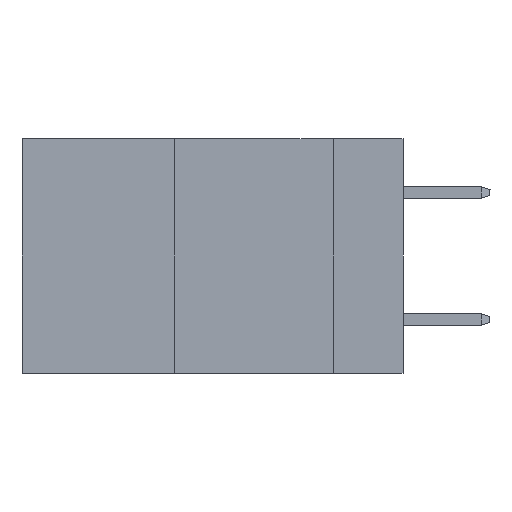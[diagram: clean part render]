
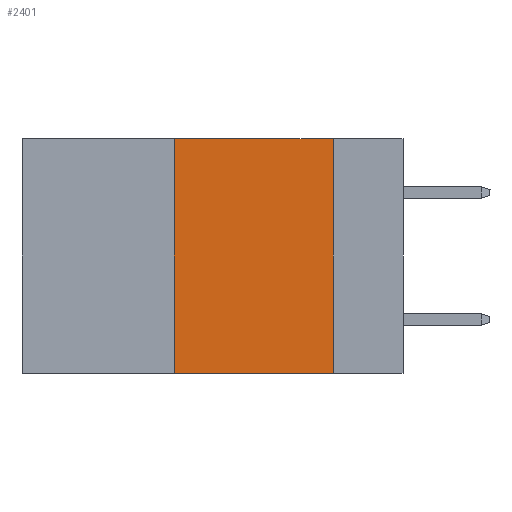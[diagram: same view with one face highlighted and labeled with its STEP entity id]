
A CAD part, left-side view. The second image highlights one B-rep face of the part: STEP entity #2401.
In plain terms, the highlighted planar face has unit normal (-1, 0, 0).
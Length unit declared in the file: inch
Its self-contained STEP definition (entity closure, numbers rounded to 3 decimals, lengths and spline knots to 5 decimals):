
#1137 = CARTESIAN_POINT ( 'NONE',  ( 0., 0.6, -0.37 ) ) ;
#1316 = CARTESIAN_POINT ( 'NONE',  ( 0., 0.36, 0. ) ) ;
#1386 = CARTESIAN_POINT ( 'NONE',  ( 0., 0.11, 0. ) ) ;
#1479 = LINE ( 'NONE', #2635, #4474 ) ;
#2294 = DIRECTION ( 'NONE',  ( 0., -1., 0. ) ) ;
#2401 = ADVANCED_FACE ( 'NONE', ( #5328 ), #10151, .F. ) ;
#2635 = CARTESIAN_POINT ( 'NONE',  ( 0., 0.6, 0. ) ) ;
#3266 = VERTEX_POINT ( 'NONE', #12657 ) ;
#3312 = LINE ( 'NONE', #9305, #13341 ) ;
#3371 = ORIENTED_EDGE ( 'NONE', *, *, #15002, .F. ) ;
#3983 = VERTEX_POINT ( 'NONE', #9104 ) ;
#4139 = DIRECTION ( 'NONE',  ( 1., 0., 0. ) ) ;
#4474 = VECTOR ( 'NONE', #13416, 39.37008 ) ;
#4542 = EDGE_LOOP ( 'NONE', ( #3371, #12261, #6507, #7021 ) ) ;
#5328 = FACE_OUTER_BOUND ( 'NONE', #4542, .T. ) ;
#5473 = VECTOR ( 'NONE', #10952, 39.37008 ) ;
#6507 = ORIENTED_EDGE ( 'NONE', *, *, #7649, .F. ) ;
#6546 = CARTESIAN_POINT ( 'NONE',  ( 0., 0.36, 0. ) ) ;
#7021 = ORIENTED_EDGE ( 'NONE', *, *, #9150, .T. ) ;
#7649 = EDGE_CURVE ( 'NONE', #3266, #13452, #12144, .T. ) ;
#8752 = EDGE_CURVE ( 'NONE', #13452, #12280, #1479, .T. ) ;
#8952 = DIRECTION ( 'NONE',  ( 0., 0., -1. ) ) ;
#9104 = CARTESIAN_POINT ( 'NONE',  ( 0., 0.11, -0.37 ) ) ;
#9150 = EDGE_CURVE ( 'NONE', #3266, #3983, #10551, .T. ) ;
#9305 = CARTESIAN_POINT ( 'NONE',  ( 0., 0.11, 0. ) ) ;
#9383 = DIRECTION ( 'NONE',  ( 0., 0., -1. ) ) ;
#10151 = PLANE ( 'NONE',  #10401 ) ;
#10401 = AXIS2_PLACEMENT_3D ( 'NONE', #14990, #4139, #8952 ) ;
#10551 = LINE ( 'NONE', #1137, #13533 ) ;
#10952 = DIRECTION ( 'NONE',  ( 0., 0., 1. ) ) ;
#12144 = LINE ( 'NONE', #1316, #5473 ) ;
#12261 = ORIENTED_EDGE ( 'NONE', *, *, #8752, .F. ) ;
#12280 = VERTEX_POINT ( 'NONE', #1386 ) ;
#12657 = CARTESIAN_POINT ( 'NONE',  ( 0., 0.36, -0.37 ) ) ;
#13341 = VECTOR ( 'NONE', #9383, 39.37008 ) ;
#13416 = DIRECTION ( 'NONE',  ( 0., -1., 0. ) ) ;
#13452 = VERTEX_POINT ( 'NONE', #6546 ) ;
#13533 = VECTOR ( 'NONE', #2294, 39.37008 ) ;
#14990 = CARTESIAN_POINT ( 'NONE',  ( 0., 0.6, 0. ) ) ;
#15002 = EDGE_CURVE ( 'NONE', #12280, #3983, #3312, .T. ) ;
